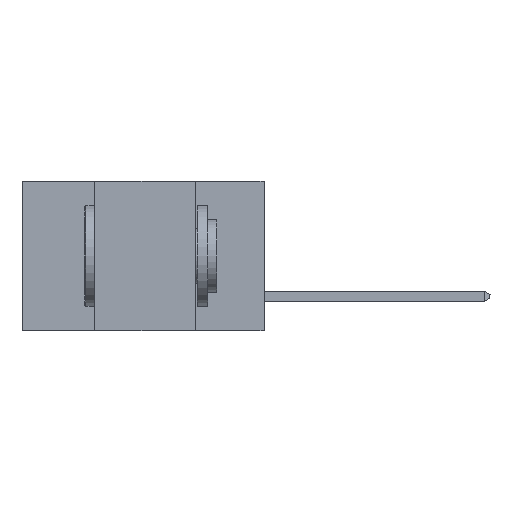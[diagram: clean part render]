
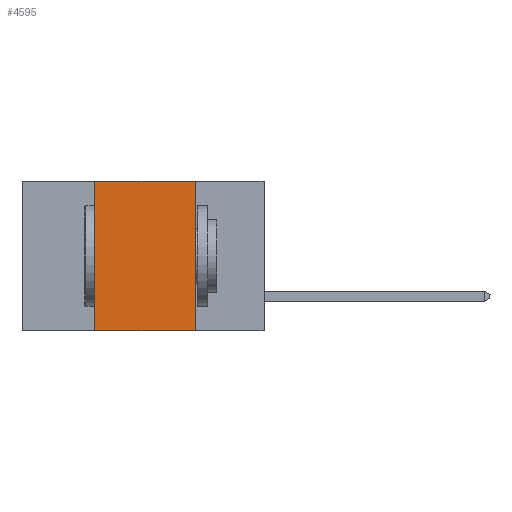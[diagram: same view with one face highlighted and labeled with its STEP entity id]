
A CAD part, left-side view. The second image highlights one B-rep face of the part: STEP entity #4595.
In plain terms, the highlighted planar face has unit normal (-1, 0, 0).
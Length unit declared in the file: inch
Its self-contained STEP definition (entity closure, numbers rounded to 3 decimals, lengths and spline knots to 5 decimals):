
#826 = CARTESIAN_POINT ( 'NONE',  ( 0., 0.17, 0. ) ) ;
#870 = FACE_OUTER_BOUND ( 'NONE', #9943, .T. ) ;
#891 = ORIENTED_EDGE ( 'NONE', *, *, #11261, .F. ) ;
#975 = PLANE ( 'NONE',  #7837 ) ;
#1981 = CARTESIAN_POINT ( 'NONE',  ( 0., 0.42, -0.37 ) ) ;
#3439 = DIRECTION ( 'NONE',  ( 0., -1., 0. ) ) ;
#3848 = ORIENTED_EDGE ( 'NONE', *, *, #19771, .T. ) ;
#4267 = VECTOR ( 'NONE', #3439, 39.37008 ) ;
#4550 = DIRECTION ( 'NONE',  ( 0., -1., 0. ) ) ;
#4595 = ADVANCED_FACE ( 'NONE', ( #870 ), #975, .F. ) ;
#4804 = VECTOR ( 'NONE', #4550, 39.37008 ) ;
#6131 = CARTESIAN_POINT ( 'NONE',  ( 0., 0.6, 0. ) ) ;
#6144 = LINE ( 'NONE', #7975, #4804 ) ;
#6756 = CARTESIAN_POINT ( 'NONE',  ( 0., 0.6, 0. ) ) ;
#7837 = AXIS2_PLACEMENT_3D ( 'NONE', #6131, #12538, #14147 ) ;
#7975 = CARTESIAN_POINT ( 'NONE',  ( 0., 0.6, -0.37 ) ) ;
#8907 = VECTOR ( 'NONE', #17354, 39.37008 ) ;
#9019 = LINE ( 'NONE', #17150, #8907 ) ;
#9943 = EDGE_LOOP ( 'NONE', ( #18443, #891, #12232, #3848 ) ) ;
#11261 = EDGE_CURVE ( 'NONE', #11468, #20167, #19614, .T. ) ;
#11468 = VERTEX_POINT ( 'NONE', #17131 ) ;
#12232 = ORIENTED_EDGE ( 'NONE', *, *, #18851, .F. ) ;
#12538 = DIRECTION ( 'NONE',  ( 1., 0., 0. ) ) ;
#14147 = DIRECTION ( 'NONE',  ( 0., 0., -1. ) ) ;
#14376 = CARTESIAN_POINT ( 'NONE',  ( 0., 0.17, -0.37 ) ) ;
#15805 = CARTESIAN_POINT ( 'NONE',  ( 0., 0.17, -0.37 ) ) ;
#16445 = VERTEX_POINT ( 'NONE', #1981 ) ;
#17131 = CARTESIAN_POINT ( 'NONE',  ( 0., 0.42, 0. ) ) ;
#17150 = CARTESIAN_POINT ( 'NONE',  ( 0., 0.42, -0.37 ) ) ;
#17354 = DIRECTION ( 'NONE',  ( 0., 0., 1. ) ) ;
#17595 = DIRECTION ( 'NONE',  ( 0., 0., -1. ) ) ;
#18329 = EDGE_CURVE ( 'NONE', #20167, #19247, #20494, .T. ) ;
#18443 = ORIENTED_EDGE ( 'NONE', *, *, #18329, .F. ) ;
#18851 = EDGE_CURVE ( 'NONE', #16445, #11468, #9019, .T. ) ;
#19247 = VERTEX_POINT ( 'NONE', #15805 ) ;
#19614 = LINE ( 'NONE', #6756, #4267 ) ;
#19771 = EDGE_CURVE ( 'NONE', #16445, #19247, #6144, .T. ) ;
#20164 = VECTOR ( 'NONE', #17595, 39.37008 ) ;
#20167 = VERTEX_POINT ( 'NONE', #826 ) ;
#20494 = LINE ( 'NONE', #14376, #20164 ) ;
